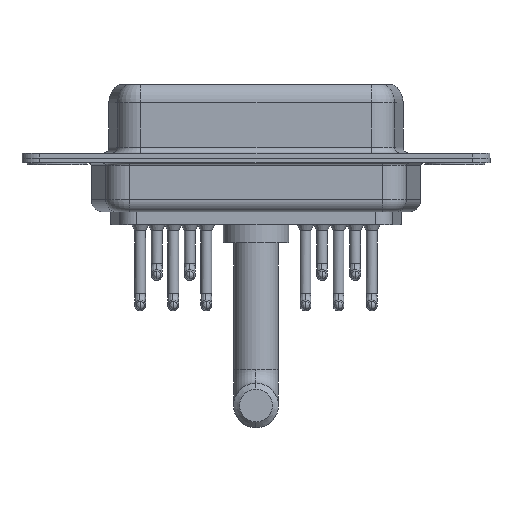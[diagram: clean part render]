
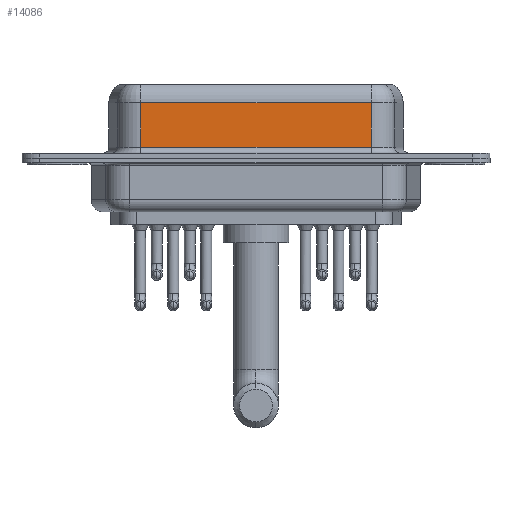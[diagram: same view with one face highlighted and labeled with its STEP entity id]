
A CAD part, front view. The second image highlights one B-rep face of the part: STEP entity #14086.
In plain terms, the highlighted planar face has unit normal (0, -1, 0).
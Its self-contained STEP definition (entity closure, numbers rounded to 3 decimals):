
#386 = AXIS2_PLACEMENT_3D ( 'NONE', #5842, #3289, #5677 ) ;
#815 = VERTEX_POINT ( 'NONE', #15840 ) ;
#1145 = CARTESIAN_POINT ( 'NONE',  ( 26.287, -3.95, 4.65 ) ) ;
#1203 = EDGE_CURVE ( 'NONE', #15843, #15956, #7200, .T. ) ;
#1398 = CARTESIAN_POINT ( 'NONE',  ( 26.287, -3.95, 0.9 ) ) ;
#2507 = LINE ( 'NONE', #1398, #11292 ) ;
#2958 = PLANE ( 'NONE',  #386 ) ;
#3103 = CARTESIAN_POINT ( 'NONE',  ( 26.287, -3.95, 6.4 ) ) ;
#3289 = DIRECTION ( 'NONE',  ( 0., 1., 0. ) ) ;
#4936 = ORIENTED_EDGE ( 'NONE', *, *, #6950, .T. ) ;
#5543 = VECTOR ( 'NONE', #10609, 1000. ) ;
#5677 = DIRECTION ( 'NONE',  ( 0., 0., 1. ) ) ;
#5842 = CARTESIAN_POINT ( 'NONE',  ( 26.287, -3.95, 6.4 ) ) ;
#5910 = CARTESIAN_POINT ( 'NONE',  ( 7.013, -3.95, 6.4 ) ) ;
#6950 = EDGE_CURVE ( 'NONE', #15956, #11590, #2507, .T. ) ;
#7200 = LINE ( 'NONE', #5910, #9922 ) ;
#8109 = ORIENTED_EDGE ( 'NONE', *, *, #14463, .T. ) ;
#8802 = CARTESIAN_POINT ( 'NONE',  ( 7.013, -3.95, 0.9 ) ) ;
#8984 = DIRECTION ( 'NONE',  ( -1., 0., 0. ) ) ;
#9657 = LINE ( 'NONE', #3103, #5543 ) ;
#9922 = VECTOR ( 'NONE', #14957, 1000. ) ;
#10609 = DIRECTION ( 'NONE',  ( 0., 0., -1. ) ) ;
#11292 = VECTOR ( 'NONE', #14456, 1000. ) ;
#11590 = VERTEX_POINT ( 'NONE', #14818 ) ;
#12309 = FACE_OUTER_BOUND ( 'NONE', #15040, .T. ) ;
#13304 = EDGE_CURVE ( 'NONE', #815, #11590, #9657, .T. ) ;
#13384 = ORIENTED_EDGE ( 'NONE', *, *, #1203, .T. ) ;
#13443 = ORIENTED_EDGE ( 'NONE', *, *, #13304, .F. ) ;
#14086 = ADVANCED_FACE ( 'NONE', ( #12309 ), #2958, .F. ) ;
#14456 = DIRECTION ( 'NONE',  ( 1., 0., 0. ) ) ;
#14463 = EDGE_CURVE ( 'NONE', #815, #15843, #16851, .T. ) ;
#14591 = VECTOR ( 'NONE', #8984, 1000. ) ;
#14640 = CARTESIAN_POINT ( 'NONE',  ( 7.013, -3.95, 4.65 ) ) ;
#14818 = CARTESIAN_POINT ( 'NONE',  ( 26.287, -3.95, 0.9 ) ) ;
#14957 = DIRECTION ( 'NONE',  ( 0., 0., -1. ) ) ;
#15040 = EDGE_LOOP ( 'NONE', ( #13443, #8109, #13384, #4936 ) ) ;
#15840 = CARTESIAN_POINT ( 'NONE',  ( 26.287, -3.95, 4.65 ) ) ;
#15843 = VERTEX_POINT ( 'NONE', #14640 ) ;
#15956 = VERTEX_POINT ( 'NONE', #8802 ) ;
#16851 = LINE ( 'NONE', #1145, #14591 ) ;
